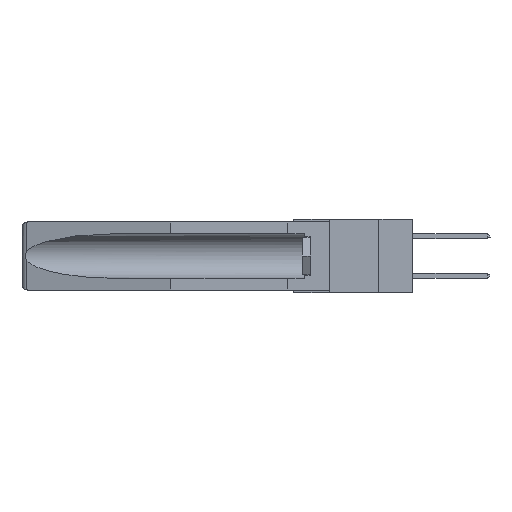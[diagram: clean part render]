
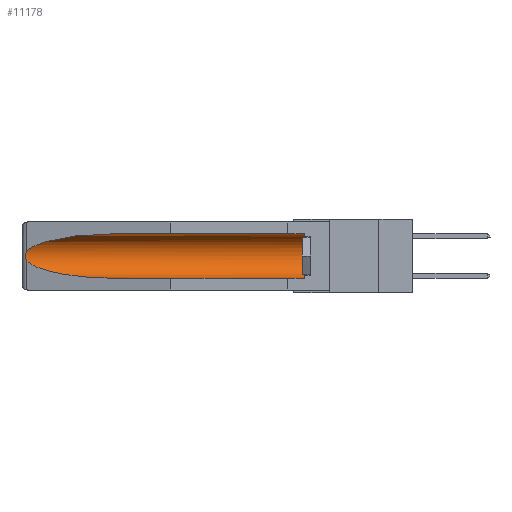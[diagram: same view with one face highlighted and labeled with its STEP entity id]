
A CAD part, left-side view. The second image highlights one B-rep face of the part: STEP entity #11178.
In plain terms, the highlighted cylindrical face has radius 2.857 mm (diameter 5.715 mm), a partial arc.
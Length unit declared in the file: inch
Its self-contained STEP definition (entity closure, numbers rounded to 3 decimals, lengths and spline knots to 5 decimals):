
#152 = B_SPLINE_CURVE_WITH_KNOTS ( 'NONE', 3,
 ( #11386, #11631, #455, #4062, #7818, #5690, #9694, #2190, #5773, #15112 ),
 .UNSPECIFIED., .F., .F.,
 ( 4, 2, 2, 2, 4 ),
 ( 0., 0.00029, 0.00058, 0.00087, 0.00117 ),
 .UNSPECIFIED. ) ;
#394 = EDGE_CURVE ( 'NONE', #7738, #10466, #12133, .T. ) ;
#455 = CARTESIAN_POINT ( 'NONE',  ( 0.26654, 1.53092, -0.15636 ) ) ;
#982 = DIRECTION ( 'NONE',  ( 0., 0., 1. ) ) ;
#1552 = DIRECTION ( 'NONE',  ( 0., -1., 0. ) ) ;
#1975 = CARTESIAN_POINT ( 'NONE',  ( 0.26537, 1.52718, -0.14972 ) ) ;
#2190 = CARTESIAN_POINT ( 'NONE',  ( 0.26655, 1.53094, -0.18657 ) ) ;
#3308 = ORIENTED_EDGE ( 'NONE', *, *, #3432, .T. ) ;
#3431 = DIRECTION ( 'NONE',  ( 0., 0., 1. ) ) ;
#3432 = EDGE_CURVE ( 'NONE', #16292, #7738, #152, .T. ) ;
#4062 = CARTESIAN_POINT ( 'NONE',  ( 0.2673, 1.5327, -0.16383 ) ) ;
#4880 = CARTESIAN_POINT ( 'NONE',  ( 0.155, 1.07973, -0.284 ) ) ;
#4980 = EDGE_CURVE ( 'NONE', #6828, #16292, #11822, .T. ) ;
#5649 = ORIENTED_EDGE ( 'NONE', *, *, #394, .T. ) ;
#5690 = CARTESIAN_POINT ( 'NONE',  ( 0.2675, 1.53308, -0.17534 ) ) ;
#5773 = CARTESIAN_POINT ( 'NONE',  ( 0.26597, 1.5296, -0.19026 ) ) ;
#6007 = AXIS2_PLACEMENT_3D ( 'NONE', #12722, #1552, #3431 ) ;
#6320 = DIRECTION ( 'NONE',  ( 0., 1., 0. ) ) ;
#6828 = VERTEX_POINT ( 'NONE', #19246 ) ;
#7242 = CARTESIAN_POINT ( 'NONE',  ( 0.155, 1.07973, -0.284 ) ) ;
#7503 = VERTEX_POINT ( 'NONE', #18793 ) ;
#7738 = VERTEX_POINT ( 'NONE', #15700 ) ;
#7818 = CARTESIAN_POINT ( 'NONE',  ( 0.2675, 1.53308, -0.16763 ) ) ;
#8168 = DIRECTION ( 'NONE',  ( 0., 1., 0. ) ) ;
#8321 = VECTOR ( 'NONE', #19640, 39.37008 ) ;
#8359 = CARTESIAN_POINT ( 'NONE',  ( 0.155, -0.30754, -0.059 ) ) ;
#9478 = CIRCLE ( 'NONE', #6007, 0.1125 ) ;
#9694 = CARTESIAN_POINT ( 'NONE',  ( 0.2673, 1.53269, -0.17917 ) ) ;
#10093 = FACE_OUTER_BOUND ( 'NONE', #12926, .T. ) ;
#10466 = VERTEX_POINT ( 'NONE', #4880 ) ;
#10957 = ORIENTED_EDGE ( 'NONE', *, *, #4980, .T. ) ;
#11178 = ADVANCED_FACE ( 'NONE', ( #10093 ), #22619, .F. ) ;
#11201 = CARTESIAN_POINT ( 'NONE',  ( 0.26537, 1.52718, -0.14972 ) ) ;
#11219 = EDGE_CURVE ( 'NONE', #18842, #10466, #18212, .T. ) ;
#11386 = CARTESIAN_POINT ( 'NONE',  ( 0.26537, 1.52718, -0.14972 ) ) ;
#11614 = EDGE_CURVE ( 'NONE', #18842, #7503, #9478, .T. ) ;
#11631 = CARTESIAN_POINT ( 'NONE',  ( 0.26597, 1.52961, -0.15275 ) ) ;
#11822 =( BOUNDED_CURVE ( )  B_SPLINE_CURVE ( 3, ( #15094, #17390, #20485, #11201 ),
 .UNSPECIFIED., .F., .F. ) 
 B_SPLINE_CURVE_WITH_KNOTS ( ( 4, 4 ),
 ( 4.71239, 6.08839 ),
 .UNSPECIFIED. ) 
 CURVE ( )  GEOMETRIC_REPRESENTATION_ITEM ( )  RATIONAL_B_SPLINE_CURVE ( ( 1., 0.848, 0.848, 1. ) ) 
 REPRESENTATION_ITEM ( '' )  );
#11984 = LINE ( 'NONE', #8359, #15748 ) ;
#12133 =( BOUNDED_CURVE ( )  B_SPLINE_CURVE ( 3, ( #20346, #16510, #18481, #7242 ),
 .UNSPECIFIED., .F., .F. ) 
 B_SPLINE_CURVE_WITH_KNOTS ( ( 4, 4 ),
 ( 0.1948, 1.5708 ),
 .UNSPECIFIED. ) 
 CURVE ( )  GEOMETRIC_REPRESENTATION_ITEM ( )  RATIONAL_B_SPLINE_CURVE ( ( 1., 0.848, 0.848, 1. ) ) 
 REPRESENTATION_ITEM ( '' )  );
#12722 = CARTESIAN_POINT ( 'NONE',  ( 0.155, 0.126, -0.1715 ) ) ;
#12735 = CARTESIAN_POINT ( 'NONE',  ( 0.155, 0.126, -0.284 ) ) ;
#12926 = EDGE_LOOP ( 'NONE', ( #10957, #3308, #5649, #16607, #21596, #17160 ) ) ;
#15094 = CARTESIAN_POINT ( 'NONE',  ( 0.155, 1.07973, -0.059 ) ) ;
#15112 = CARTESIAN_POINT ( 'NONE',  ( 0.26537, 1.52718, -0.19328 ) ) ;
#15700 = CARTESIAN_POINT ( 'NONE',  ( 0.26537, 1.52718, -0.19328 ) ) ;
#15748 = VECTOR ( 'NONE', #6320, 39.37008 ) ;
#16292 = VERTEX_POINT ( 'NONE', #1975 ) ;
#16510 = CARTESIAN_POINT ( 'NONE',  ( 0.25451, 1.48313, -0.24835 ) ) ;
#16607 = ORIENTED_EDGE ( 'NONE', *, *, #11219, .F. ) ;
#17160 = ORIENTED_EDGE ( 'NONE', *, *, #22238, .T. ) ;
#17390 = CARTESIAN_POINT ( 'NONE',  ( 0.21114, 1.30732, -0.059 ) ) ;
#18002 = AXIS2_PLACEMENT_3D ( 'NONE', #23325, #8168, #982 ) ;
#18212 = LINE ( 'NONE', #21355, #8321 ) ;
#18481 = CARTESIAN_POINT ( 'NONE',  ( 0.21114, 1.30732, -0.284 ) ) ;
#18793 = CARTESIAN_POINT ( 'NONE',  ( 0.155, 0.126, -0.059 ) ) ;
#18842 = VERTEX_POINT ( 'NONE', #12735 ) ;
#19246 = CARTESIAN_POINT ( 'NONE',  ( 0.155, 1.07973, -0.059 ) ) ;
#19640 = DIRECTION ( 'NONE',  ( 0., 1., 0. ) ) ;
#20346 = CARTESIAN_POINT ( 'NONE',  ( 0.26537, 1.52718, -0.19328 ) ) ;
#20485 = CARTESIAN_POINT ( 'NONE',  ( 0.25451, 1.48313, -0.09465 ) ) ;
#21355 = CARTESIAN_POINT ( 'NONE',  ( 0.155, -0.30754, -0.284 ) ) ;
#21596 = ORIENTED_EDGE ( 'NONE', *, *, #11614, .T. ) ;
#22238 = EDGE_CURVE ( 'NONE', #7503, #6828, #11984, .T. ) ;
#22619 = CYLINDRICAL_SURFACE ( 'NONE', #18002, 0.1125 ) ;
#23325 = CARTESIAN_POINT ( 'NONE',  ( 0.155, -0.30754, -0.1715 ) ) ;
